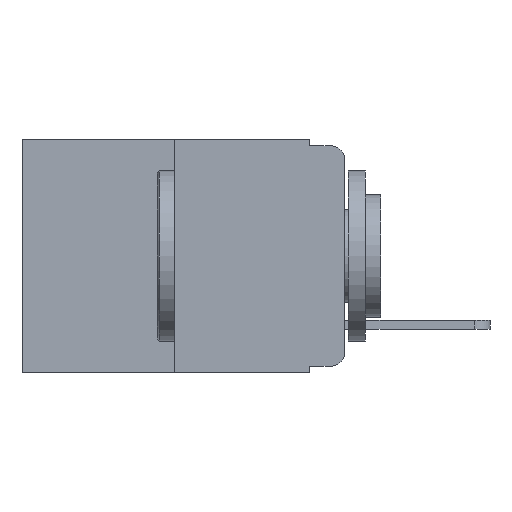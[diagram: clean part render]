
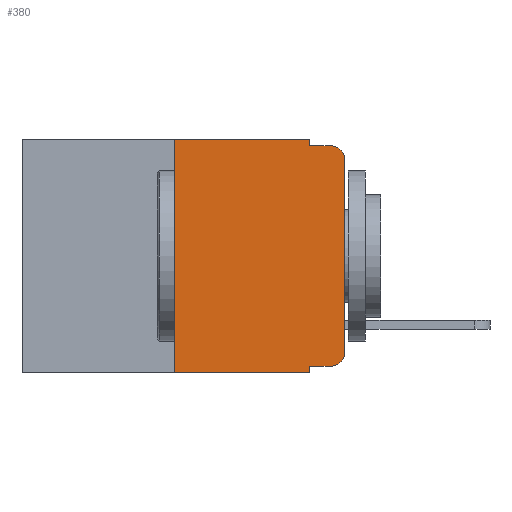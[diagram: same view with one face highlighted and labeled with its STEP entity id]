
A CAD part, left-side view. The second image highlights one B-rep face of the part: STEP entity #380.
In plain terms, the highlighted planar face has unit normal (-1, 0, 0).
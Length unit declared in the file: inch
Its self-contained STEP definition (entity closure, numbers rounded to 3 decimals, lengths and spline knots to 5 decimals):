
#380 = ADVANCED_FACE ( 'NONE', ( #5327 ), #12038, .F. ) ;
#508 = DIRECTION ( 'NONE',  ( -1., 0., 0. ) ) ;
#574 = DIRECTION ( 'NONE',  ( 0., 0., -1. ) ) ;
#753 = CARTESIAN_POINT ( 'NONE',  ( 0., 0.02, -0.03 ) ) ;
#775 = EDGE_CURVE ( 'NONE', #5868, #7521, #12396, .T. ) ;
#989 = CARTESIAN_POINT ( 'NONE',  ( 0., 0.02, -0.01 ) ) ;
#1449 = EDGE_CURVE ( 'NONE', #7479, #3346, #7160, .T. ) ;
#1454 = EDGE_CURVE ( 'NONE', #3346, #6492, #6726, .T. ) ;
#1476 = EDGE_CURVE ( 'NONE', #2277, #6492, #6934, .T. ) ;
#1559 = EDGE_CURVE ( 'NONE', #10634, #2277, #4283, .T. ) ;
#1564 = EDGE_CURVE ( 'NONE', #5868, #4649, #4101, .T. ) ;
#1587 = EDGE_CURVE ( 'NONE', #3062, #7521, #3683, .T. ) ;
#1614 = EDGE_CURVE ( 'NONE', #3062, #4609, #3696, .T. ) ;
#1641 = EDGE_CURVE ( 'NONE', #4609, #7479, #3434, .T. ) ;
#2051 = DIRECTION ( 'NONE',  ( 0., 0., -1. ) ) ;
#2143 = DIRECTION ( 'NONE',  ( 0., -1., 0. ) ) ;
#2212 = CARTESIAN_POINT ( 'NONE',  ( 0., 0.051, -0.01 ) ) ;
#2277 = VERTEX_POINT ( 'NONE', #7891 ) ;
#2535 = CARTESIAN_POINT ( 'NONE',  ( 0., 0.051, -0.333 ) ) ;
#2612 = DIRECTION ( 'NONE',  ( 0., 0., 1. ) ) ;
#3062 = VERTEX_POINT ( 'NONE', #12071 ) ;
#3346 = VERTEX_POINT ( 'NONE', #12661 ) ;
#3434 = CIRCLE ( 'NONE', #12584, 0.02 ) ;
#3497 = VECTOR ( 'NONE', #12235, 39.37008 ) ;
#3654 = VECTOR ( 'NONE', #2051, 39.37008 ) ;
#3683 = LINE ( 'NONE', #10585, #3654 ) ;
#3696 = LINE ( 'NONE', #2535, #3497 ) ;
#4101 = LINE ( 'NONE', #4925, #4128 ) ;
#4128 = VECTOR ( 'NONE', #11492, 39.37008 ) ;
#4283 = LINE ( 'NONE', #10101, #4638 ) ;
#4609 = VERTEX_POINT ( 'NONE', #12115 ) ;
#4638 = VECTOR ( 'NONE', #13363, 39.37008 ) ;
#4649 = VERTEX_POINT ( 'NONE', #11435 ) ;
#4925 = CARTESIAN_POINT ( 'NONE',  ( 0., 0.25, 0. ) ) ;
#5327 = FACE_OUTER_BOUND ( 'NONE', #12549, .T. ) ;
#5371 = CARTESIAN_POINT ( 'NONE',  ( 0., 0., 0. ) ) ;
#5520 = VECTOR ( 'NONE', #2143, 39.37008 ) ;
#5651 = DIRECTION ( 'NONE',  ( 0., -1., 0. ) ) ;
#5715 = CARTESIAN_POINT ( 'NONE',  ( 0., 0.473, 0. ) ) ;
#5868 = VERTEX_POINT ( 'NONE', #9471 ) ;
#6492 = VERTEX_POINT ( 'NONE', #989 ) ;
#6607 = VECTOR ( 'NONE', #2612, 39.37008 ) ;
#6726 = CIRCLE ( 'NONE', #7322, 0.02 ) ;
#6934 = LINE ( 'NONE', #2212, #5520 ) ;
#6993 = AXIS2_PLACEMENT_3D ( 'NONE', #9802, #9164, #11102 ) ;
#7160 = LINE ( 'NONE', #5371, #6607 ) ;
#7322 = AXIS2_PLACEMENT_3D ( 'NONE', #753, #508, #574 ) ;
#7396 = DIRECTION ( 'NONE',  ( -1., 0., 0. ) ) ;
#7446 = CARTESIAN_POINT ( 'NONE',  ( 0., 0.02, -0.313 ) ) ;
#7479 = VERTEX_POINT ( 'NONE', #11143 ) ;
#7521 = VERTEX_POINT ( 'NONE', #10410 ) ;
#7891 = CARTESIAN_POINT ( 'NONE',  ( 0., 0.051, -0.01 ) ) ;
#8386 = LINE ( 'NONE', #5715, #10581 ) ;
#8811 = ORIENTED_EDGE ( 'NONE', *, *, #1449, .T. ) ;
#8821 = ORIENTED_EDGE ( 'NONE', *, *, #1454, .T. ) ;
#9127 = ORIENTED_EDGE ( 'NONE', *, *, #1476, .F. ) ;
#9164 = DIRECTION ( 'NONE',  ( 1., 0., 0. ) ) ;
#9352 = ORIENTED_EDGE ( 'NONE', *, *, #1559, .F. ) ;
#9411 = ORIENTED_EDGE ( 'NONE', *, *, #12451, .F. ) ;
#9471 = CARTESIAN_POINT ( 'NONE',  ( 0., 0.25, -0.343 ) ) ;
#9802 = CARTESIAN_POINT ( 'NONE',  ( 0., 0.473, 0. ) ) ;
#10068 = ORIENTED_EDGE ( 'NONE', *, *, #1564, .F. ) ;
#10101 = CARTESIAN_POINT ( 'NONE',  ( 0., 0.051, 0. ) ) ;
#10128 = ORIENTED_EDGE ( 'NONE', *, *, #775, .T. ) ;
#10263 = VECTOR ( 'NONE', #11943, 39.37008 ) ;
#10410 = CARTESIAN_POINT ( 'NONE',  ( 0., 0.051, -0.343 ) ) ;
#10581 = VECTOR ( 'NONE', #5651, 39.37008 ) ;
#10585 = CARTESIAN_POINT ( 'NONE',  ( 0., 0.051, 0. ) ) ;
#10634 = VERTEX_POINT ( 'NONE', #11096 ) ;
#11096 = CARTESIAN_POINT ( 'NONE',  ( 0., 0.051, 0. ) ) ;
#11102 = DIRECTION ( 'NONE',  ( 0., 0., -1. ) ) ;
#11143 = CARTESIAN_POINT ( 'NONE',  ( 0., 0., -0.313 ) ) ;
#11188 = DIRECTION ( 'NONE',  ( 0., 0., -1. ) ) ;
#11424 = CARTESIAN_POINT ( 'NONE',  ( 0., 0.473, -0.343 ) ) ;
#11435 = CARTESIAN_POINT ( 'NONE',  ( 0., 0.25, 0. ) ) ;
#11492 = DIRECTION ( 'NONE',  ( 0., 0., 1. ) ) ;
#11943 = DIRECTION ( 'NONE',  ( 0., -1., 0. ) ) ;
#12038 = PLANE ( 'NONE',  #6993 ) ;
#12071 = CARTESIAN_POINT ( 'NONE',  ( 0., 0.051, -0.333 ) ) ;
#12115 = CARTESIAN_POINT ( 'NONE',  ( 0., 0.02, -0.333 ) ) ;
#12129 = ORIENTED_EDGE ( 'NONE', *, *, #1587, .F. ) ;
#12167 = ORIENTED_EDGE ( 'NONE', *, *, #1614, .T. ) ;
#12235 = DIRECTION ( 'NONE',  ( 0., -1., 0. ) ) ;
#12250 = ORIENTED_EDGE ( 'NONE', *, *, #1641, .T. ) ;
#12396 = LINE ( 'NONE', #11424, #10263 ) ;
#12451 = EDGE_CURVE ( 'NONE', #4649, #10634, #8386, .T. ) ;
#12549 = EDGE_LOOP ( 'NONE', ( #8811, #8821, #9127, #9352, #9411, #10068, #10128, #12129, #12167, #12250 ) ) ;
#12584 = AXIS2_PLACEMENT_3D ( 'NONE', #7446, #7396, #11188 ) ;
#12661 = CARTESIAN_POINT ( 'NONE',  ( 0., 0., -0.03 ) ) ;
#13363 = DIRECTION ( 'NONE',  ( 0., 0., -1. ) ) ;
